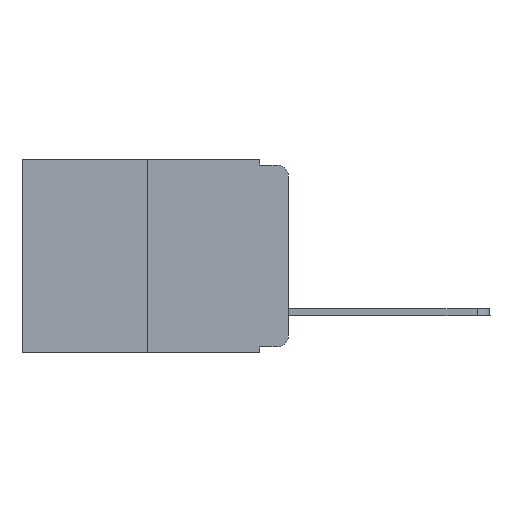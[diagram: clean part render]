
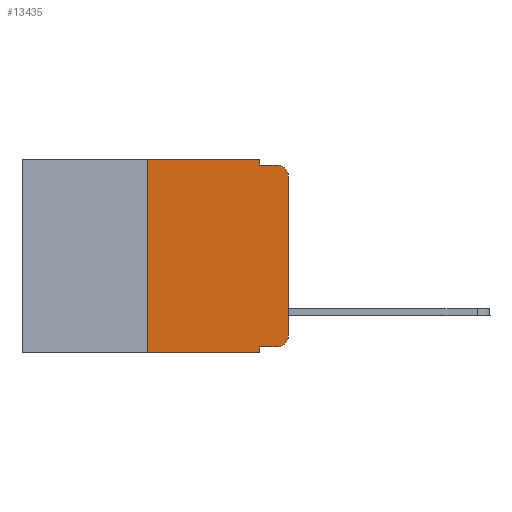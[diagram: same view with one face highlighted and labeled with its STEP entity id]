
A CAD part, left-side view. The second image highlights one B-rep face of the part: STEP entity #13435.
In plain terms, the highlighted planar face has unit normal (-1, 0, 0).
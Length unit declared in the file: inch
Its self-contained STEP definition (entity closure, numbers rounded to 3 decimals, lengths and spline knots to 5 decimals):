
#7 = DIRECTION ( 'NONE',  ( 0., 0., 1. ) ) ;
#179 = CIRCLE ( 'NONE', #12763, 0.02 ) ;
#244 = VERTEX_POINT ( 'NONE', #3468 ) ;
#1137 = DIRECTION ( 'NONE',  ( 0., 0., -1. ) ) ;
#1259 = DIRECTION ( 'NONE',  ( 0., 0., 1. ) ) ;
#1467 = LINE ( 'NONE', #21216, #7827 ) ;
#1531 = CARTESIAN_POINT ( 'NONE',  ( 0., 0.25, -0.343 ) ) ;
#1609 = EDGE_CURVE ( 'NONE', #23561, #23424, #179, .T. ) ;
#1640 = ORIENTED_EDGE ( 'NONE', *, *, #21123, .T. ) ;
#1960 = VERTEX_POINT ( 'NONE', #11561 ) ;
#2301 = DIRECTION ( 'NONE',  ( 0., -1., 0. ) ) ;
#2396 = CARTESIAN_POINT ( 'NONE',  ( 0., 0.02, -0.01 ) ) ;
#2448 = ORIENTED_EDGE ( 'NONE', *, *, #20476, .F. ) ;
#2763 = FACE_OUTER_BOUND ( 'NONE', #3799, .T. ) ;
#3344 = VERTEX_POINT ( 'NONE', #7995 ) ;
#3468 = CARTESIAN_POINT ( 'NONE',  ( 0., 0.25, 0. ) ) ;
#3799 = EDGE_LOOP ( 'NONE', ( #21864, #8118, #2448, #6716, #6128, #8894, #7357, #10550, #1640, #24220 ) ) ;
#4438 = PLANE ( 'NONE',  #18334 ) ;
#5286 = LINE ( 'NONE', #12821, #20032 ) ;
#6128 = ORIENTED_EDGE ( 'NONE', *, *, #14541, .F. ) ;
#6232 = EDGE_CURVE ( 'NONE', #3344, #11857, #11411, .T. ) ;
#6295 = VECTOR ( 'NONE', #20383, 39.37008 ) ;
#6595 = CIRCLE ( 'NONE', #11694, 0.02 ) ;
#6716 = ORIENTED_EDGE ( 'NONE', *, *, #19502, .F. ) ;
#7252 = CARTESIAN_POINT ( 'NONE',  ( 0., 0.473, -0.343 ) ) ;
#7357 = ORIENTED_EDGE ( 'NONE', *, *, #8468, .T. ) ;
#7583 = LINE ( 'NONE', #14087, #19897 ) ;
#7595 = DIRECTION ( 'NONE',  ( 0., -1., 0. ) ) ;
#7782 = CARTESIAN_POINT ( 'NONE',  ( 0., 0.02, -0.313 ) ) ;
#7827 = VECTOR ( 'NONE', #7, 39.37008 ) ;
#7995 = CARTESIAN_POINT ( 'NONE',  ( 0., 0.051, -0.333 ) ) ;
#8118 = ORIENTED_EDGE ( 'NONE', *, *, #1609, .T. ) ;
#8468 = EDGE_CURVE ( 'NONE', #24424, #11857, #22546, .T. ) ;
#8493 = CARTESIAN_POINT ( 'NONE',  ( 0., 0.051, -0.01 ) ) ;
#8894 = ORIENTED_EDGE ( 'NONE', *, *, #10003, .F. ) ;
#9206 = DIRECTION ( 'NONE',  ( 0., 0., -1. ) ) ;
#9862 = DIRECTION ( 'NONE',  ( 0., 0., -1. ) ) ;
#10003 = EDGE_CURVE ( 'NONE', #24424, #244, #5286, .T. ) ;
#10550 = ORIENTED_EDGE ( 'NONE', *, *, #6232, .F. ) ;
#11183 = VECTOR ( 'NONE', #7595, 39.37008 ) ;
#11411 = LINE ( 'NONE', #22138, #6295 ) ;
#11561 = CARTESIAN_POINT ( 'NONE',  ( 0., 0.02, -0.333 ) ) ;
#11595 = CARTESIAN_POINT ( 'NONE',  ( 0., 0., -0.313 ) ) ;
#11694 = AXIS2_PLACEMENT_3D ( 'NONE', #7782, #15311, #9862 ) ;
#11855 = VECTOR ( 'NONE', #1137, 39.37008 ) ;
#11857 = VERTEX_POINT ( 'NONE', #15926 ) ;
#12090 = VECTOR ( 'NONE', #14286, 39.37008 ) ;
#12295 = VERTEX_POINT ( 'NONE', #18635 ) ;
#12454 = LINE ( 'NONE', #18233, #11855 ) ;
#12763 = AXIS2_PLACEMENT_3D ( 'NONE', #20724, #24620, #9206 ) ;
#12821 = CARTESIAN_POINT ( 'NONE',  ( 0., 0.25, 0. ) ) ;
#13435 = ADVANCED_FACE ( 'NONE', ( #2763 ), #4438, .F. ) ;
#14087 = CARTESIAN_POINT ( 'NONE',  ( 0., 0.051, -0.333 ) ) ;
#14242 = DIRECTION ( 'NONE',  ( 0., 0., -1. ) ) ;
#14286 = DIRECTION ( 'NONE',  ( 0., -1., 0. ) ) ;
#14381 = VECTOR ( 'NONE', #23276, 39.37008 ) ;
#14530 = VERTEX_POINT ( 'NONE', #11595 ) ;
#14541 = EDGE_CURVE ( 'NONE', #244, #19960, #15998, .T. ) ;
#15311 = DIRECTION ( 'NONE',  ( -1., 0., 0. ) ) ;
#15926 = CARTESIAN_POINT ( 'NONE',  ( 0., 0.051, -0.343 ) ) ;
#15933 = CARTESIAN_POINT ( 'NONE',  ( 0., 0.473, 0. ) ) ;
#15998 = LINE ( 'NONE', #17157, #11183 ) ;
#16215 = CARTESIAN_POINT ( 'NONE',  ( 0., 0., -0.03 ) ) ;
#17157 = CARTESIAN_POINT ( 'NONE',  ( 0., 0.473, 0. ) ) ;
#17517 = LINE ( 'NONE', #8493, #12090 ) ;
#18233 = CARTESIAN_POINT ( 'NONE',  ( 0., 0.051, 0. ) ) ;
#18334 = AXIS2_PLACEMENT_3D ( 'NONE', #15933, #21748, #14242 ) ;
#18635 = CARTESIAN_POINT ( 'NONE',  ( 0., 0.051, -0.01 ) ) ;
#19502 = EDGE_CURVE ( 'NONE', #19960, #12295, #12454, .T. ) ;
#19897 = VECTOR ( 'NONE', #2301, 39.37008 ) ;
#19960 = VERTEX_POINT ( 'NONE', #23931 ) ;
#20032 = VECTOR ( 'NONE', #1259, 39.37008 ) ;
#20383 = DIRECTION ( 'NONE',  ( 0., 0., -1. ) ) ;
#20476 = EDGE_CURVE ( 'NONE', #12295, #23424, #17517, .T. ) ;
#20724 = CARTESIAN_POINT ( 'NONE',  ( 0., 0.02, -0.03 ) ) ;
#21123 = EDGE_CURVE ( 'NONE', #3344, #1960, #7583, .T. ) ;
#21216 = CARTESIAN_POINT ( 'NONE',  ( 0., 0., 0. ) ) ;
#21748 = DIRECTION ( 'NONE',  ( 1., 0., 0. ) ) ;
#21864 = ORIENTED_EDGE ( 'NONE', *, *, #22153, .T. ) ;
#22138 = CARTESIAN_POINT ( 'NONE',  ( 0., 0.051, 0. ) ) ;
#22153 = EDGE_CURVE ( 'NONE', #14530, #23561, #1467, .T. ) ;
#22546 = LINE ( 'NONE', #7252, #14381 ) ;
#22746 = EDGE_CURVE ( 'NONE', #1960, #14530, #6595, .T. ) ;
#23276 = DIRECTION ( 'NONE',  ( 0., -1., 0. ) ) ;
#23424 = VERTEX_POINT ( 'NONE', #2396 ) ;
#23561 = VERTEX_POINT ( 'NONE', #16215 ) ;
#23931 = CARTESIAN_POINT ( 'NONE',  ( 0., 0.051, 0. ) ) ;
#24220 = ORIENTED_EDGE ( 'NONE', *, *, #22746, .T. ) ;
#24424 = VERTEX_POINT ( 'NONE', #1531 ) ;
#24620 = DIRECTION ( 'NONE',  ( -1., 0., 0. ) ) ;
